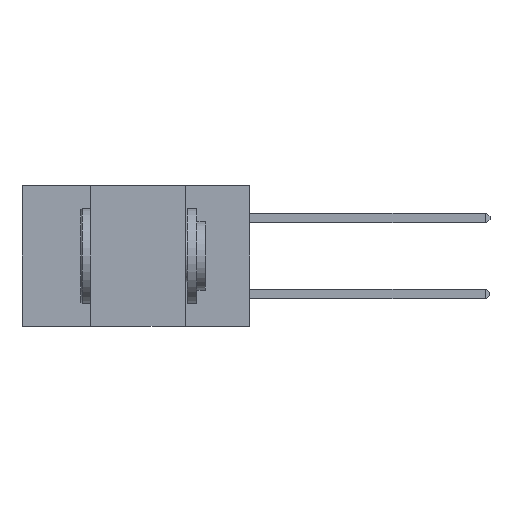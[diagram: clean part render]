
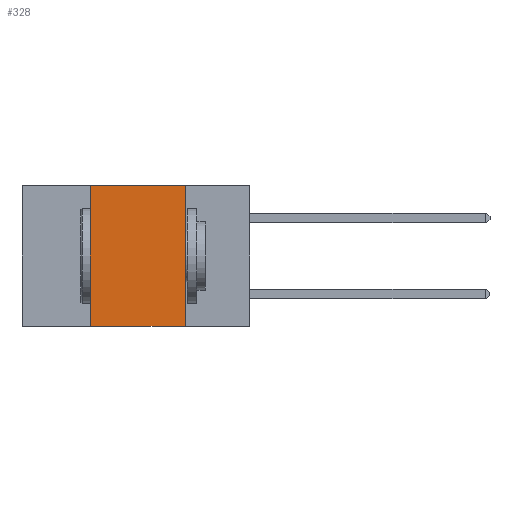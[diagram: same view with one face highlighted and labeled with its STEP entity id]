
A CAD part, left-side view. The second image highlights one B-rep face of the part: STEP entity #328.
In plain terms, the highlighted planar face has unit normal (-1, 0, 0).
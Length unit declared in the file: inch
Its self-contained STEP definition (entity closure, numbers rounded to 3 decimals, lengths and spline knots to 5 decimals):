
#197 = LINE ( 'NONE', #4098, #8181 ) ;
#328 = ADVANCED_FACE ( 'NONE', ( #6331 ), #8226, .F. ) ;
#702 = VERTEX_POINT ( 'NONE', #6728 ) ;
#1417 = LINE ( 'NONE', #4039, #9005 ) ;
#1600 = VERTEX_POINT ( 'NONE', #5954 ) ;
#1833 = EDGE_CURVE ( 'NONE', #6196, #702, #1417, .T. ) ;
#2005 = AXIS2_PLACEMENT_3D ( 'NONE', #4293, #2643, #2844 ) ;
#2418 = ORIENTED_EDGE ( 'NONE', *, *, #1833, .T. ) ;
#2643 = DIRECTION ( 'NONE',  ( 1., 0., 0. ) ) ;
#2794 = EDGE_LOOP ( 'NONE', ( #3502, #4024, #7589, #2418 ) ) ;
#2844 = DIRECTION ( 'NONE',  ( 0., 0., -1. ) ) ;
#3339 = LINE ( 'NONE', #7934, #6788 ) ;
#3502 = ORIENTED_EDGE ( 'NONE', *, *, #4056, .F. ) ;
#3915 = DIRECTION ( 'NONE',  ( 0., 0., -1. ) ) ;
#4024 = ORIENTED_EDGE ( 'NONE', *, *, #9523, .F. ) ;
#4032 = DIRECTION ( 'NONE',  ( 0., -1., 0. ) ) ;
#4039 = CARTESIAN_POINT ( 'NONE',  ( 0., 0.6, -0.37 ) ) ;
#4056 = EDGE_CURVE ( 'NONE', #5448, #702, #197, .T. ) ;
#4098 = CARTESIAN_POINT ( 'NONE',  ( 0., 0.17, 0. ) ) ;
#4293 = CARTESIAN_POINT ( 'NONE',  ( 0., 0.6, 0. ) ) ;
#4580 = CARTESIAN_POINT ( 'NONE',  ( 0., 0.6, 0. ) ) ;
#5107 = VECTOR ( 'NONE', #9374, 39.37008 ) ;
#5183 = EDGE_CURVE ( 'NONE', #6196, #1600, #3339, .T. ) ;
#5448 = VERTEX_POINT ( 'NONE', #9203 ) ;
#5888 = CARTESIAN_POINT ( 'NONE',  ( 0., 0.42, -0.37 ) ) ;
#5954 = CARTESIAN_POINT ( 'NONE',  ( 0., 0.42, 0. ) ) ;
#6196 = VERTEX_POINT ( 'NONE', #5888 ) ;
#6331 = FACE_OUTER_BOUND ( 'NONE', #2794, .T. ) ;
#6728 = CARTESIAN_POINT ( 'NONE',  ( 0., 0.17, -0.37 ) ) ;
#6788 = VECTOR ( 'NONE', #7789, 39.37008 ) ;
#7589 = ORIENTED_EDGE ( 'NONE', *, *, #5183, .F. ) ;
#7789 = DIRECTION ( 'NONE',  ( 0., 0., 1. ) ) ;
#7934 = CARTESIAN_POINT ( 'NONE',  ( 0., 0.42, 0. ) ) ;
#8181 = VECTOR ( 'NONE', #3915, 39.37008 ) ;
#8226 = PLANE ( 'NONE',  #2005 ) ;
#8778 = LINE ( 'NONE', #4580, #5107 ) ;
#9005 = VECTOR ( 'NONE', #4032, 39.37008 ) ;
#9203 = CARTESIAN_POINT ( 'NONE',  ( 0., 0.17, 0. ) ) ;
#9374 = DIRECTION ( 'NONE',  ( 0., -1., 0. ) ) ;
#9523 = EDGE_CURVE ( 'NONE', #1600, #5448, #8778, .T. ) ;
